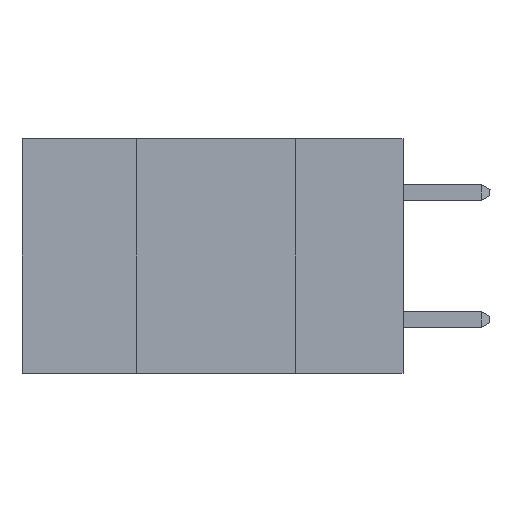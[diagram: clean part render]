
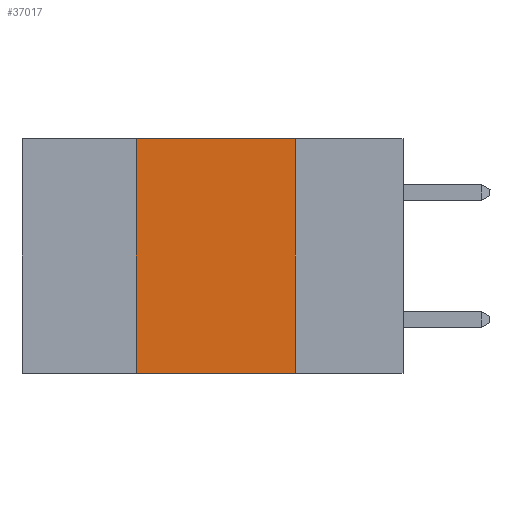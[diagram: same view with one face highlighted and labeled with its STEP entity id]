
A CAD part, left-side view. The second image highlights one B-rep face of the part: STEP entity #37017.
In plain terms, the highlighted planar face has unit normal (-1, 0, 0).
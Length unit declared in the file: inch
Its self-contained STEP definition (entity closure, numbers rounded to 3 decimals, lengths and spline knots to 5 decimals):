
#684 = CARTESIAN_POINT ( 'NONE',  ( 0., 0.17, 0. ) ) ;
#1116 = EDGE_CURVE ( 'NONE', #21436, #30501, #34213, .T. ) ;
#4294 = VECTOR ( 'NONE', #29227, 39.37008 ) ;
#4708 = DIRECTION ( 'NONE',  ( 0., 0., -1. ) ) ;
#5403 = ORIENTED_EDGE ( 'NONE', *, *, #32467, .T. ) ;
#10059 = VECTOR ( 'NONE', #25541, 39.37008 ) ;
#10480 = CARTESIAN_POINT ( 'NONE',  ( 0., 0.42, 0. ) ) ;
#10990 = LINE ( 'NONE', #33764, #15199 ) ;
#11598 = EDGE_CURVE ( 'NONE', #30501, #29970, #10990, .T. ) ;
#13777 = VECTOR ( 'NONE', #36167, 39.37008 ) ;
#14379 = LINE ( 'NONE', #37918, #4294 ) ;
#15199 = VECTOR ( 'NONE', #22169, 39.37008 ) ;
#15751 = ORIENTED_EDGE ( 'NONE', *, *, #38013, .F. ) ;
#16514 = EDGE_LOOP ( 'NONE', ( #15751, #35085, #24462, #5403 ) ) ;
#19755 = FACE_OUTER_BOUND ( 'NONE', #16514, .T. ) ;
#21323 = LINE ( 'NONE', #684, #13777 ) ;
#21436 = VERTEX_POINT ( 'NONE', #33528 ) ;
#22169 = DIRECTION ( 'NONE',  ( 0., -1., 0. ) ) ;
#22834 = CARTESIAN_POINT ( 'NONE',  ( 0., 0.6, 0. ) ) ;
#22881 = CARTESIAN_POINT ( 'NONE',  ( 0., 0.17, 0. ) ) ;
#23224 = PLANE ( 'NONE',  #32804 ) ;
#24462 = ORIENTED_EDGE ( 'NONE', *, *, #1116, .F. ) ;
#25541 = DIRECTION ( 'NONE',  ( 0., 0., 1. ) ) ;
#28808 = DIRECTION ( 'NONE',  ( 1., 0., 0. ) ) ;
#29191 = CARTESIAN_POINT ( 'NONE',  ( 0., 0.42, 0. ) ) ;
#29227 = DIRECTION ( 'NONE',  ( 0., -1., 0. ) ) ;
#29273 = VERTEX_POINT ( 'NONE', #36248 ) ;
#29970 = VERTEX_POINT ( 'NONE', #22881 ) ;
#30501 = VERTEX_POINT ( 'NONE', #29191 ) ;
#32467 = EDGE_CURVE ( 'NONE', #21436, #29273, #14379, .T. ) ;
#32804 = AXIS2_PLACEMENT_3D ( 'NONE', #22834, #28808, #4708 ) ;
#33528 = CARTESIAN_POINT ( 'NONE',  ( 0., 0.42, -0.37 ) ) ;
#33764 = CARTESIAN_POINT ( 'NONE',  ( 0., 0.6, 0. ) ) ;
#34213 = LINE ( 'NONE', #10480, #10059 ) ;
#35085 = ORIENTED_EDGE ( 'NONE', *, *, #11598, .F. ) ;
#36167 = DIRECTION ( 'NONE',  ( 0., 0., -1. ) ) ;
#36248 = CARTESIAN_POINT ( 'NONE',  ( 0., 0.17, -0.37 ) ) ;
#37017 = ADVANCED_FACE ( 'NONE', ( #19755 ), #23224, .F. ) ;
#37918 = CARTESIAN_POINT ( 'NONE',  ( 0., 0.6, -0.37 ) ) ;
#38013 = EDGE_CURVE ( 'NONE', #29970, #29273, #21323, .T. ) ;
